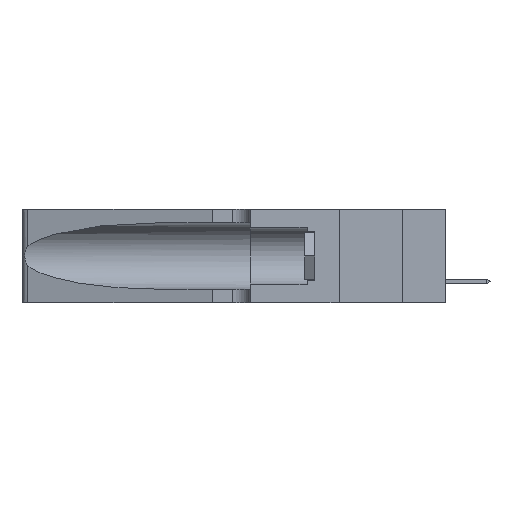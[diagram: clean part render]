
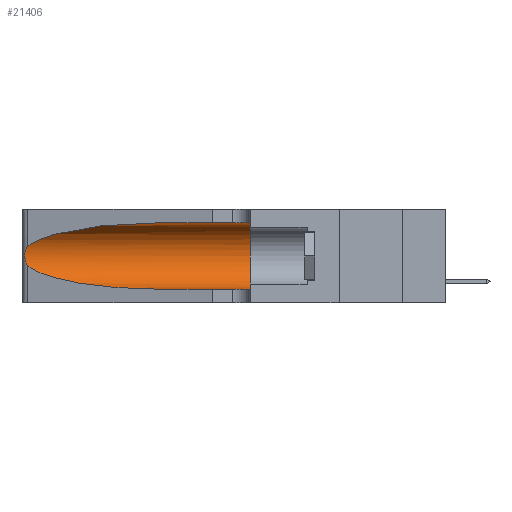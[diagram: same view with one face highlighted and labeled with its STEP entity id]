
A CAD part, left-side view. The second image highlights one B-rep face of the part: STEP entity #21406.
In plain terms, the highlighted cylindrical face has radius 3.308 mm (diameter 6.617 mm), a partial arc.
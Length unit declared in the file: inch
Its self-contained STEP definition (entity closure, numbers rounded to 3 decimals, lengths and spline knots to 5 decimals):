
#495 = CARTESIAN_POINT ( 'NONE',  ( 0.25487, 1.22718, 0.14631 ) ) ;
#1055 = VERTEX_POINT ( 'NONE', #13720 ) ;
#2203 = CARTESIAN_POINT ( 'NONE',  ( 0.1305, 0.72297, 0.31525 ) ) ;
#2874 = VERTEX_POINT ( 'NONE', #37161 ) ;
#3206 = AXIS2_PLACEMENT_3D ( 'NONE', #40635, #9971, #9264 ) ;
#3498 = FACE_OUTER_BOUND ( 'NONE', #22012, .T. ) ;
#4050 = ORIENTED_EDGE ( 'NONE', *, *, #34022, .T. ) ;
#4656 = CARTESIAN_POINT ( 'NONE',  ( 0.25639, 1.23186, 0.15144 ) ) ;
#4810 = CARTESIAN_POINT ( 'NONE',  ( 0.25789, 1.23486, 0.15765 ) ) ;
#4979 = CARTESIAN_POINT ( 'NONE',  ( 0.25555, 1.22993, 0.14849 ) ) ;
#5905 = AXIS2_PLACEMENT_3D ( 'NONE', #46498, #8391, #12002 ) ;
#6703 = LINE ( 'NONE', #24568, #15166 ) ;
#6764 = ORIENTED_EDGE ( 'NONE', *, *, #48327, .T. ) ;
#8307 = EDGE_CURVE ( 'NONE', #28754, #2874, #40675, .T. ) ;
#8391 = DIRECTION ( 'NONE',  ( 0., -1., 0. ) ) ;
#9264 = DIRECTION ( 'NONE',  ( 0., 0., 1. ) ) ;
#9971 = DIRECTION ( 'NONE',  ( 0., 1., 0. ) ) ;
#12002 = DIRECTION ( 'NONE',  ( 0., 0., -1. ) ) ;
#12045 = CARTESIAN_POINT ( 'NONE',  ( 0.26075, 1.23896, 0.178 ) ) ;
#12452 = VERTEX_POINT ( 'NONE', #36645 ) ;
#13720 = CARTESIAN_POINT ( 'NONE',  ( 0.1305, 0.72297, 0.05475 ) ) ;
#14898 = ORIENTED_EDGE ( 'NONE', *, *, #34507, .T. ) ;
#15166 = VECTOR ( 'NONE', #16974, 39.37008 ) ;
#15192 = EDGE_CURVE ( 'NONE', #19514, #1055, #24995, .T. ) ;
#15899 = CARTESIAN_POINT ( 'NONE',  ( 0.25487, 1.22718, 0.14631 ) ) ;
#15949 = EDGE_CURVE ( 'NONE', #2874, #12452, #43244, .T. ) ;
#16100 = CARTESIAN_POINT ( 'NONE',  ( 0.2373, 1.15595, 0.08982 ) ) ;
#16926 = B_SPLINE_CURVE_WITH_KNOTS ( 'NONE', 3,
 ( #20408, #47470, #28054, #27740, #35186, #23993, #35700, #12045, #35530, #35356, #4810, #4656, #4979, #15899 ),
 .UNSPECIFIED., .F., .F.,
 ( 4, 2, 2, 2, 2, 2, 4 ),
 ( 0., 0.00027, 0.00053, 0.00107, 0.0016, 0.00187, 0.00214 ),
 .UNSPECIFIED. ) ;
#16974 = DIRECTION ( 'NONE',  ( 0., -1., 0. ) ) ;
#18790 = ORIENTED_EDGE ( 'NONE', *, *, #15192, .T. ) ;
#18923 = ORIENTED_EDGE ( 'NONE', *, *, #8307, .F. ) ;
#19514 = VERTEX_POINT ( 'NONE', #47482 ) ;
#20408 = CARTESIAN_POINT ( 'NONE',  ( 0.25487, 1.22718, 0.22369 ) ) ;
#21277 =( BOUNDED_CURVE ( )  B_SPLINE_CURVE ( 3, ( #2203, #48360, #29825, #32842 ),
 .UNSPECIFIED., .F., .F. ) 
 B_SPLINE_CURVE_WITH_KNOTS ( ( 4, 4 ),
 ( 1.5708, 2.84003 ),
 .UNSPECIFIED. ) 
 CURVE ( )  GEOMETRIC_REPRESENTATION_ITEM ( )  RATIONAL_B_SPLINE_CURVE ( ( 1., 0.87, 0.87, 1. ) ) 
 REPRESENTATION_ITEM ( '' )  );
#21406 = ADVANCED_FACE ( 'NONE', ( #3498 ), #48865, .F. ) ;
#22012 = EDGE_LOOP ( 'NONE', ( #4050, #6764, #18790, #14898, #30426, #18923 ) ) ;
#23993 = CARTESIAN_POINT ( 'NONE',  ( 0.26018, 1.23835, 0.19895 ) ) ;
#24568 = CARTESIAN_POINT ( 'NONE',  ( 0.1305, 1.61858, 0.05475 ) ) ;
#24995 =( BOUNDED_CURVE ( )  B_SPLINE_CURVE ( 3, ( #495, #16100, #39177, #27930 ),
 .UNSPECIFIED., .F., .F. ) 
 B_SPLINE_CURVE_WITH_KNOTS ( ( 4, 4 ),
 ( 3.44316, 4.71239 ),
 .UNSPECIFIED. ) 
 CURVE ( )  GEOMETRIC_REPRESENTATION_ITEM ( )  RATIONAL_B_SPLINE_CURVE ( ( 1., 0.87, 0.87, 1. ) ) 
 REPRESENTATION_ITEM ( '' )  );
#25320 = CARTESIAN_POINT ( 'NONE',  ( 0.1305, 0.72297, 0.31525 ) ) ;
#25444 = CARTESIAN_POINT ( 'NONE',  ( 0.25487, 1.22718, 0.22369 ) ) ;
#27740 = CARTESIAN_POINT ( 'NONE',  ( 0.25787, 1.23484, 0.2124 ) ) ;
#27930 = CARTESIAN_POINT ( 'NONE',  ( 0.1305, 0.72297, 0.05475 ) ) ;
#28054 = CARTESIAN_POINT ( 'NONE',  ( 0.25639, 1.23184, 0.21858 ) ) ;
#28754 = VERTEX_POINT ( 'NONE', #25320 ) ;
#29825 = CARTESIAN_POINT ( 'NONE',  ( 0.2373, 1.15595, 0.28018 ) ) ;
#30426 = ORIENTED_EDGE ( 'NONE', *, *, #15949, .F. ) ;
#32842 = CARTESIAN_POINT ( 'NONE',  ( 0.25487, 1.22718, 0.22369 ) ) ;
#34022 = EDGE_CURVE ( 'NONE', #28754, #47920, #21277, .T. ) ;
#34507 = EDGE_CURVE ( 'NONE', #1055, #12452, #6703, .T. ) ;
#35186 = CARTESIAN_POINT ( 'NONE',  ( 0.25854, 1.2359, 0.20912 ) ) ;
#35356 = CARTESIAN_POINT ( 'NONE',  ( 0.25856, 1.23593, 0.16098 ) ) ;
#35530 = CARTESIAN_POINT ( 'NONE',  ( 0.26017, 1.23833, 0.17102 ) ) ;
#35700 = CARTESIAN_POINT ( 'NONE',  ( 0.26075, 1.23896, 0.19203 ) ) ;
#36645 = CARTESIAN_POINT ( 'NONE',  ( 0.1305, 0.35, 0.05475 ) ) ;
#37161 = CARTESIAN_POINT ( 'NONE',  ( 0.1305, 0.35, 0.31525 ) ) ;
#39177 = CARTESIAN_POINT ( 'NONE',  ( 0.18966, 0.96281, 0.05475 ) ) ;
#40635 = CARTESIAN_POINT ( 'NONE',  ( 0.1305, 0.35, 0.185 ) ) ;
#40675 = LINE ( 'NONE', #42270, #43044 ) ;
#42270 = CARTESIAN_POINT ( 'NONE',  ( 0.1305, 1.61858, 0.31525 ) ) ;
#43044 = VECTOR ( 'NONE', #45295, 39.37008 ) ;
#43244 = CIRCLE ( 'NONE', #3206, 0.13025 ) ;
#45295 = DIRECTION ( 'NONE',  ( 0., -1., 0. ) ) ;
#46498 = CARTESIAN_POINT ( 'NONE',  ( 0.1305, 1.61858, 0.185 ) ) ;
#47470 = CARTESIAN_POINT ( 'NONE',  ( 0.25555, 1.22994, 0.2215 ) ) ;
#47482 = CARTESIAN_POINT ( 'NONE',  ( 0.25487, 1.22718, 0.14631 ) ) ;
#47920 = VERTEX_POINT ( 'NONE', #25444 ) ;
#48327 = EDGE_CURVE ( 'NONE', #47920, #19514, #16926, .T. ) ;
#48360 = CARTESIAN_POINT ( 'NONE',  ( 0.18966, 0.96281, 0.31525 ) ) ;
#48865 = CYLINDRICAL_SURFACE ( 'NONE', #5905, 0.13025 ) ;
